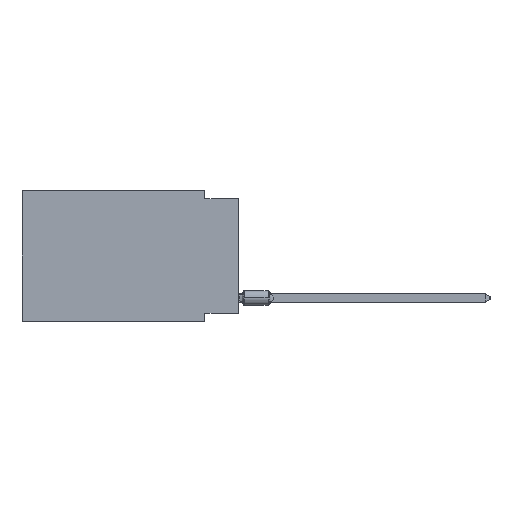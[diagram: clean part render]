
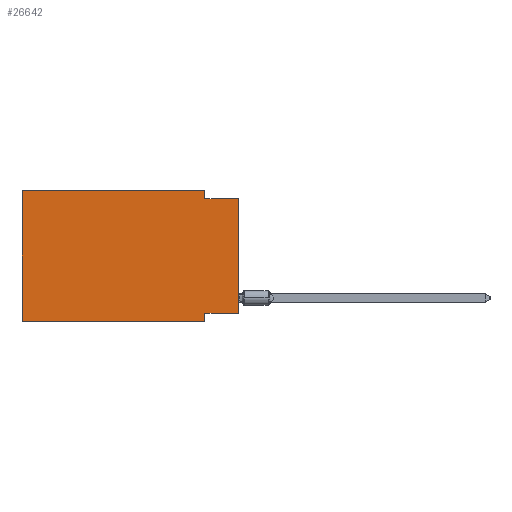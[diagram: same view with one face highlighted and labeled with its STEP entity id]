
A CAD part, left-side view. The second image highlights one B-rep face of the part: STEP entity #26642.
In plain terms, the highlighted planar face has unit normal (-1, 0, 0).
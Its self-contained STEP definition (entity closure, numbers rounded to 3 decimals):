
#3294 = EDGE_CURVE ( 'NONE', #5865, #12651, #54387, .T. ) ;
#4072 = DIRECTION ( 'NONE',  ( 0., -1., 0. ) ) ;
#4149 = ORIENTED_EDGE ( 'NONE', *, *, #25463, .F. ) ;
#4796 = LINE ( 'NONE', #23600, #7991 ) ;
#5046 = LINE ( 'NONE', #22492, #52049 ) ;
#5319 = DIRECTION ( 'NONE',  ( 0., -1., 0. ) ) ;
#5546 = AXIS2_PLACEMENT_3D ( 'NONE', #26158, #43618, #49045 ) ;
#5607 = LINE ( 'NONE', #48858, #36865 ) ;
#5865 = VERTEX_POINT ( 'NONE', #47266 ) ;
#6908 = VERTEX_POINT ( 'NONE', #28313 ) ;
#7991 = VECTOR ( 'NONE', #44312, 1000. ) ;
#9564 = PLANE ( 'NONE',  #5546 ) ;
#10287 = EDGE_CURVE ( 'NONE', #6908, #15715, #16223, .T. ) ;
#10429 = CARTESIAN_POINT ( 'NONE',  ( 0., 2.54, -9.271 ) ) ;
#10587 = DIRECTION ( 'NONE',  ( 0., 0., -1. ) ) ;
#10680 = VECTOR ( 'NONE', #51142, 1000. ) ;
#11727 = LINE ( 'NONE', #19739, #16299 ) ;
#12651 = VERTEX_POINT ( 'NONE', #22564 ) ;
#13829 = CARTESIAN_POINT ( 'NONE',  ( 0., 2.54, 0. ) ) ;
#15715 = VERTEX_POINT ( 'NONE', #22367 ) ;
#15798 = ORIENTED_EDGE ( 'NONE', *, *, #3294, .F. ) ;
#16223 = LINE ( 'NONE', #33675, #10680 ) ;
#16299 = VECTOR ( 'NONE', #46094, 1000. ) ;
#16570 = ORIENTED_EDGE ( 'NONE', *, *, #54835, .T. ) ;
#18468 = CARTESIAN_POINT ( 'NONE',  ( 0., 0., -9.271 ) ) ;
#18498 = VECTOR ( 'NONE', #4072, 1000. ) ;
#19739 = CARTESIAN_POINT ( 'NONE',  ( 0., 0., -9.271 ) ) ;
#22367 = CARTESIAN_POINT ( 'NONE',  ( 0., 2.54, -9.906 ) ) ;
#22406 = EDGE_CURVE ( 'NONE', #25222, #15715, #5046, .T. ) ;
#22492 = CARTESIAN_POINT ( 'NONE',  ( 0., 2.54, -9.906 ) ) ;
#22564 = CARTESIAN_POINT ( 'NONE',  ( 0., 2.54, -0.635 ) ) ;
#23600 = CARTESIAN_POINT ( 'NONE',  ( 0., 0., 0. ) ) ;
#25222 = VERTEX_POINT ( 'NONE', #10429 ) ;
#25463 = EDGE_CURVE ( 'NONE', #35252, #5865, #30680, .T. ) ;
#26158 = CARTESIAN_POINT ( 'NONE',  ( 0., 16.383, 0. ) ) ;
#26193 = EDGE_CURVE ( 'NONE', #6908, #35252, #33218, .T. ) ;
#26642 = ADVANCED_FACE ( 'NONE', ( #53366 ), #9564, .F. ) ;
#26809 = DIRECTION ( 'NONE',  ( 0., 0., -1. ) ) ;
#26831 = CARTESIAN_POINT ( 'NONE',  ( 0., 0., -0.635 ) ) ;
#28313 = CARTESIAN_POINT ( 'NONE',  ( 0., 16.383, -9.906 ) ) ;
#30680 = LINE ( 'NONE', #47884, #18498 ) ;
#33218 = LINE ( 'NONE', #50694, #41160 ) ;
#33675 = CARTESIAN_POINT ( 'NONE',  ( 0., 16.383, -9.906 ) ) ;
#34643 = VERTEX_POINT ( 'NONE', #18468 ) ;
#35252 = VERTEX_POINT ( 'NONE', #51317 ) ;
#36335 = ORIENTED_EDGE ( 'NONE', *, *, #55843, .F. ) ;
#36796 = VECTOR ( 'NONE', #10587, 1000. ) ;
#36865 = VECTOR ( 'NONE', #5319, 1000. ) ;
#39828 = ORIENTED_EDGE ( 'NONE', *, *, #10287, .T. ) ;
#41160 = VECTOR ( 'NONE', #55536, 1000. ) ;
#41868 = ORIENTED_EDGE ( 'NONE', *, *, #49990, .F. ) ;
#43442 = ORIENTED_EDGE ( 'NONE', *, *, #26193, .F. ) ;
#43618 = DIRECTION ( 'NONE',  ( 1., 0., 0. ) ) ;
#43939 = ORIENTED_EDGE ( 'NONE', *, *, #22406, .F. ) ;
#44312 = DIRECTION ( 'NONE',  ( 0., 0., 1. ) ) ;
#46094 = DIRECTION ( 'NONE',  ( 0., 1., 0. ) ) ;
#46588 = EDGE_LOOP ( 'NONE', ( #16570, #41868, #15798, #4149, #43442, #39828, #43939, #36335 ) ) ;
#47266 = CARTESIAN_POINT ( 'NONE',  ( 0., 2.54, 0. ) ) ;
#47884 = CARTESIAN_POINT ( 'NONE',  ( 0., 16.383, 0. ) ) ;
#48858 = CARTESIAN_POINT ( 'NONE',  ( 0., 0., -0.635 ) ) ;
#49045 = DIRECTION ( 'NONE',  ( 0., 0., -1. ) ) ;
#49990 = EDGE_CURVE ( 'NONE', #12651, #53100, #5607, .T. ) ;
#50694 = CARTESIAN_POINT ( 'NONE',  ( 0., 16.383, 0. ) ) ;
#51142 = DIRECTION ( 'NONE',  ( 0., -1., 0. ) ) ;
#51317 = CARTESIAN_POINT ( 'NONE',  ( 0., 16.383, 0. ) ) ;
#52049 = VECTOR ( 'NONE', #26809, 1000. ) ;
#53100 = VERTEX_POINT ( 'NONE', #26831 ) ;
#53366 = FACE_OUTER_BOUND ( 'NONE', #46588, .T. ) ;
#54387 = LINE ( 'NONE', #13829, #36796 ) ;
#54835 = EDGE_CURVE ( 'NONE', #34643, #53100, #4796, .T. ) ;
#55536 = DIRECTION ( 'NONE',  ( 0., 0., 1. ) ) ;
#55843 = EDGE_CURVE ( 'NONE', #34643, #25222, #11727, .T. ) ;
